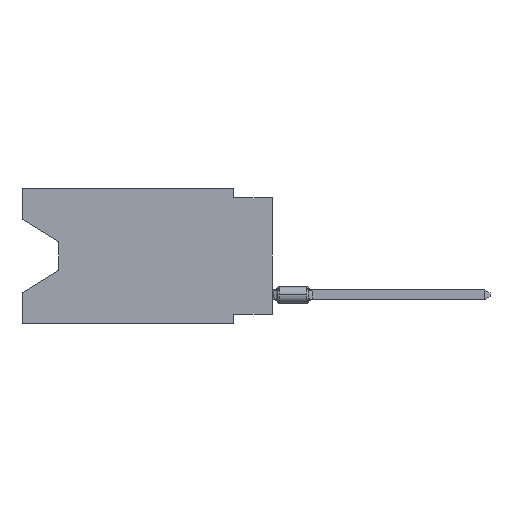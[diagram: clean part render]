
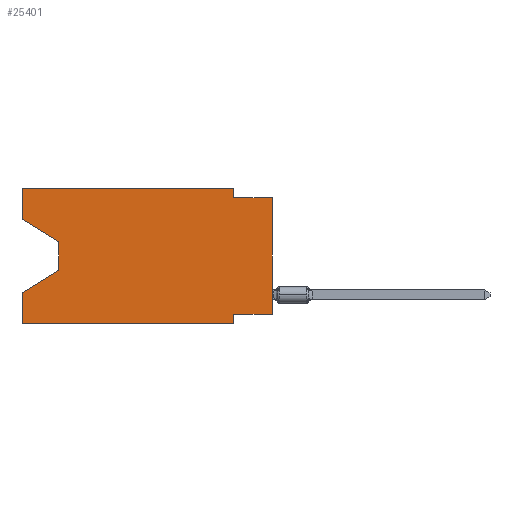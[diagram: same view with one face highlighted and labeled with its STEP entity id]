
A CAD part, left-side view. The second image highlights one B-rep face of the part: STEP entity #25401.
In plain terms, the highlighted planar face has unit normal (-1, 0, 0).
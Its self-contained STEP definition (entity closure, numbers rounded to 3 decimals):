
#7 = VERTEX_POINT ( 'NONE', #11791 ) ;
#626 = ORIENTED_EDGE ( 'NONE', *, *, #6556, .T. ) ;
#746 = CARTESIAN_POINT ( 'NONE',  ( 0., 0., -8.255 ) ) ;
#767 = VECTOR ( 'NONE', #13235, 1000. ) ;
#1174 = LINE ( 'NONE', #9169, #10807 ) ;
#1716 = DIRECTION ( 'NONE',  ( 0., 0., -1. ) ) ;
#1905 = DIRECTION ( 'NONE',  ( 0., 0., -1. ) ) ;
#2300 = CARTESIAN_POINT ( 'NONE',  ( 0., 2.54, -0.635 ) ) ;
#3096 = VECTOR ( 'NONE', #17737, 1000. ) ;
#3549 = VECTOR ( 'NONE', #12858, 1000. ) ;
#4408 = CARTESIAN_POINT ( 'NONE',  ( 0., 2.54, 0. ) ) ;
#4534 = DIRECTION ( 'NONE',  ( 0., 0., 1. ) ) ;
#4893 = LINE ( 'NONE', #16659, #3549 ) ;
#5149 = VERTEX_POINT ( 'NONE', #12830 ) ;
#5181 = ORIENTED_EDGE ( 'NONE', *, *, #14700, .F. ) ;
#5281 = CARTESIAN_POINT ( 'NONE',  ( 0., 16.383, 0. ) ) ;
#5372 = VERTEX_POINT ( 'NONE', #24064 ) ;
#5799 = LINE ( 'NONE', #15318, #20882 ) ;
#6137 = CARTESIAN_POINT ( 'NONE',  ( 0., 0., -0.635 ) ) ;
#6319 = CARTESIAN_POINT ( 'NONE',  ( 0., 2.54, 0. ) ) ;
#6556 = EDGE_CURVE ( 'NONE', #5149, #7196, #10081, .T. ) ;
#6938 = ORIENTED_EDGE ( 'NONE', *, *, #20749, .T. ) ;
#7072 = VERTEX_POINT ( 'NONE', #2300 ) ;
#7196 = VERTEX_POINT ( 'NONE', #11147 ) ;
#7750 = FACE_OUTER_BOUND ( 'NONE', #23997, .T. ) ;
#8183 = ORIENTED_EDGE ( 'NONE', *, *, #23270, .F. ) ;
#8419 = VERTEX_POINT ( 'NONE', #15657 ) ;
#8517 = VECTOR ( 'NONE', #24070, 1000. ) ;
#8751 = ORIENTED_EDGE ( 'NONE', *, *, #13546, .T. ) ;
#8815 = EDGE_CURVE ( 'NONE', #8419, #9767, #23608, .T. ) ;
#9169 = CARTESIAN_POINT ( 'NONE',  ( 0., 16.383, -8.89 ) ) ;
#9499 = VECTOR ( 'NONE', #20260, 1000. ) ;
#9756 = CARTESIAN_POINT ( 'NONE',  ( 0., 16.383, 0. ) ) ;
#9767 = VERTEX_POINT ( 'NONE', #14222 ) ;
#10081 = LINE ( 'NONE', #20027, #8517 ) ;
#10666 = EDGE_CURVE ( 'NONE', #7072, #15803, #18273, .T. ) ;
#10807 = VECTOR ( 'NONE', #18171, 1000. ) ;
#10843 = VERTEX_POINT ( 'NONE', #9756 ) ;
#11147 = CARTESIAN_POINT ( 'NONE',  ( 0., 13.97, -3.505 ) ) ;
#11791 = CARTESIAN_POINT ( 'NONE',  ( 0., 2.54, -8.255 ) ) ;
#11833 = LINE ( 'NONE', #23334, #17873 ) ;
#11918 = ORIENTED_EDGE ( 'NONE', *, *, #18327, .F. ) ;
#12015 = CARTESIAN_POINT ( 'NONE',  ( 0., 0., 0. ) ) ;
#12109 = LINE ( 'NONE', #12611, #20279 ) ;
#12611 = CARTESIAN_POINT ( 'NONE',  ( 0., 16.383, 0. ) ) ;
#12624 = CARTESIAN_POINT ( 'NONE',  ( 0., 0., -0.635 ) ) ;
#12830 = CARTESIAN_POINT ( 'NONE',  ( 0., 16.383, -2.038 ) ) ;
#12858 = DIRECTION ( 'NONE',  ( 0., 0., -1. ) ) ;
#13078 = EDGE_CURVE ( 'NONE', #10843, #13220, #23167, .T. ) ;
#13220 = VERTEX_POINT ( 'NONE', #6319 ) ;
#13235 = DIRECTION ( 'NONE',  ( 0., -1., 0. ) ) ;
#13546 = EDGE_CURVE ( 'NONE', #20804, #15544, #1174, .T. ) ;
#14095 = EDGE_CURVE ( 'NONE', #5372, #15803, #24043, .T. ) ;
#14200 = LINE ( 'NONE', #4408, #24096 ) ;
#14222 = CARTESIAN_POINT ( 'NONE',  ( 0., 16.383, -6.852 ) ) ;
#14700 = EDGE_CURVE ( 'NONE', #20804, #9767, #5799, .T. ) ;
#15184 = CARTESIAN_POINT ( 'NONE',  ( 0., 16.383, 0. ) ) ;
#15318 = CARTESIAN_POINT ( 'NONE',  ( 0., 16.383, 0. ) ) ;
#15445 = PLANE ( 'NONE',  #25799 ) ;
#15544 = VERTEX_POINT ( 'NONE', #17756 ) ;
#15657 = CARTESIAN_POINT ( 'NONE',  ( 0., 13.97, -5.385 ) ) ;
#15803 = VERTEX_POINT ( 'NONE', #12624 ) ;
#15929 = DIRECTION ( 'NONE',  ( 0., 0., 1. ) ) ;
#15936 = ORIENTED_EDGE ( 'NONE', *, *, #22242, .F. ) ;
#16412 = DIRECTION ( 'NONE',  ( 0., 0., -1. ) ) ;
#16659 = CARTESIAN_POINT ( 'NONE',  ( 0., 2.54, -8.89 ) ) ;
#17593 = ORIENTED_EDGE ( 'NONE', *, *, #10666, .F. ) ;
#17737 = DIRECTION ( 'NONE',  ( 0., 0.855, -0.519 ) ) ;
#17756 = CARTESIAN_POINT ( 'NONE',  ( 0., 2.54, -8.89 ) ) ;
#17873 = VECTOR ( 'NONE', #1905, 1000. ) ;
#18112 = CARTESIAN_POINT ( 'NONE',  ( 0., 16.383, -8.89 ) ) ;
#18171 = DIRECTION ( 'NONE',  ( 0., -1., 0. ) ) ;
#18273 = LINE ( 'NONE', #6137, #19432 ) ;
#18327 = EDGE_CURVE ( 'NONE', #5372, #7, #22467, .T. ) ;
#18736 = ORIENTED_EDGE ( 'NONE', *, *, #24754, .F. ) ;
#19249 = DIRECTION ( 'NONE',  ( 1., 0., 0. ) ) ;
#19291 = ORIENTED_EDGE ( 'NONE', *, *, #8815, .T. ) ;
#19432 = VECTOR ( 'NONE', #22198, 1000. ) ;
#19642 = DIRECTION ( 'NONE',  ( 0., 0., 1. ) ) ;
#20027 = CARTESIAN_POINT ( 'NONE',  ( 0., 16.383, -2.038 ) ) ;
#20260 = DIRECTION ( 'NONE',  ( 0., 1., 0. ) ) ;
#20279 = VECTOR ( 'NONE', #4534, 1000. ) ;
#20749 = EDGE_CURVE ( 'NONE', #7196, #8419, #11833, .T. ) ;
#20804 = VERTEX_POINT ( 'NONE', #18112 ) ;
#20882 = VECTOR ( 'NONE', #19642, 1000. ) ;
#21324 = ORIENTED_EDGE ( 'NONE', *, *, #13078, .F. ) ;
#21660 = CARTESIAN_POINT ( 'NONE',  ( 0., 13.97, -5.385 ) ) ;
#21716 = VECTOR ( 'NONE', #15929, 1000. ) ;
#21964 = ORIENTED_EDGE ( 'NONE', *, *, #14095, .T. ) ;
#22198 = DIRECTION ( 'NONE',  ( 0., -1., 0. ) ) ;
#22242 = EDGE_CURVE ( 'NONE', #7, #15544, #4893, .T. ) ;
#22467 = LINE ( 'NONE', #746, #9499 ) ;
#23167 = LINE ( 'NONE', #5281, #767 ) ;
#23270 = EDGE_CURVE ( 'NONE', #5149, #10843, #12109, .T. ) ;
#23334 = CARTESIAN_POINT ( 'NONE',  ( 0., 13.97, -3.505 ) ) ;
#23608 = LINE ( 'NONE', #21660, #3096 ) ;
#23997 = EDGE_LOOP ( 'NONE', ( #626, #6938, #19291, #5181, #8751, #15936, #11918, #21964, #17593, #18736, #21324, #8183 ) ) ;
#24043 = LINE ( 'NONE', #12015, #21716 ) ;
#24064 = CARTESIAN_POINT ( 'NONE',  ( 0., 0., -8.255 ) ) ;
#24070 = DIRECTION ( 'NONE',  ( 0., -0.855, -0.519 ) ) ;
#24096 = VECTOR ( 'NONE', #16412, 1000. ) ;
#24754 = EDGE_CURVE ( 'NONE', #13220, #7072, #14200, .T. ) ;
#25401 = ADVANCED_FACE ( 'NONE', ( #7750 ), #15445, .F. ) ;
#25799 = AXIS2_PLACEMENT_3D ( 'NONE', #15184, #19249, #1716 ) ;
